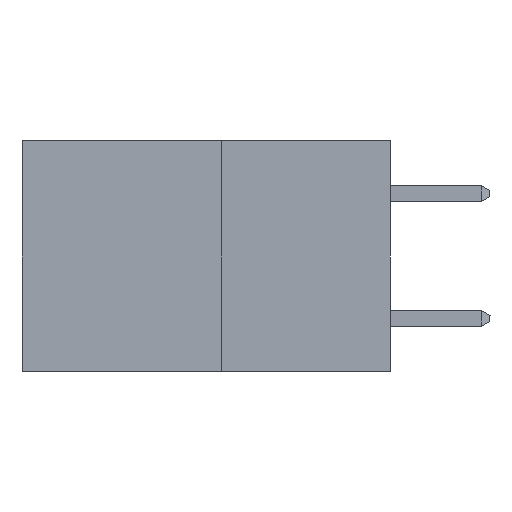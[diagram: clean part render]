
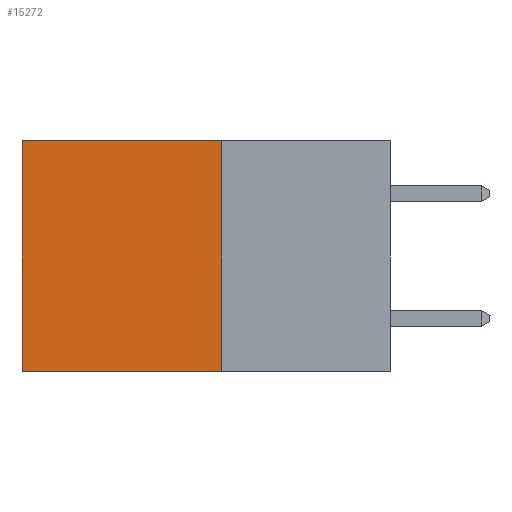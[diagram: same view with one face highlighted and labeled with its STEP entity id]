
A CAD part, left-side view. The second image highlights one B-rep face of the part: STEP entity #15272.
In plain terms, the highlighted planar face has unit normal (-1, 0, 0).
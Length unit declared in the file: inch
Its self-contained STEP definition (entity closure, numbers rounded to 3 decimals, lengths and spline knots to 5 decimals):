
#1228 = VERTEX_POINT ( 'NONE', #15493 ) ;
#1375 = PLANE ( 'NONE',  #30467 ) ;
#1493 = DIRECTION ( 'NONE',  ( 1., 0., 0. ) ) ;
#1712 = VECTOR ( 'NONE', #8613, 39.37008 ) ;
#1733 = VECTOR ( 'NONE', #33003, 39.37008 ) ;
#2395 = CARTESIAN_POINT ( 'NONE',  ( 0.277, 0.59, -0.37 ) ) ;
#2786 = VERTEX_POINT ( 'NONE', #28604 ) ;
#5936 = VECTOR ( 'NONE', #17146, 39.37008 ) ;
#6020 = CARTESIAN_POINT ( 'NONE',  ( 0.277, 0.27, -0.37 ) ) ;
#6703 = LINE ( 'NONE', #16378, #32387 ) ;
#7818 = ORIENTED_EDGE ( 'NONE', *, *, #26788, .F. ) ;
#8156 = ORIENTED_EDGE ( 'NONE', *, *, #24488, .F. ) ;
#8613 = DIRECTION ( 'NONE',  ( 0., 0., -1. ) ) ;
#10356 = ORIENTED_EDGE ( 'NONE', *, *, #28336, .T. ) ;
#12945 = ORIENTED_EDGE ( 'NONE', *, *, #30673, .T. ) ;
#12955 = CARTESIAN_POINT ( 'NONE',  ( 0.277, 0.59, -0.37 ) ) ;
#14595 = CARTESIAN_POINT ( 'NONE',  ( 0.277, 0.27, -0.37 ) ) ;
#14860 = EDGE_LOOP ( 'NONE', ( #12945, #7818, #8156, #10356 ) ) ;
#15272 = ADVANCED_FACE ( 'NONE', ( #21255 ), #1375, .F. ) ;
#15493 = CARTESIAN_POINT ( 'NONE',  ( 0.277, 0.27, 0. ) ) ;
#16360 = VERTEX_POINT ( 'NONE', #12955 ) ;
#16378 = CARTESIAN_POINT ( 'NONE',  ( 0.277, 0.27, 0. ) ) ;
#16700 = CARTESIAN_POINT ( 'NONE',  ( 0.277, 0.27, -0.37 ) ) ;
#17146 = DIRECTION ( 'NONE',  ( 0., 1., 0. ) ) ;
#18817 = VERTEX_POINT ( 'NONE', #19926 ) ;
#19293 = DIRECTION ( 'NONE',  ( 0., 0., -1. ) ) ;
#19463 = LINE ( 'NONE', #14595, #5936 ) ;
#19926 = CARTESIAN_POINT ( 'NONE',  ( 0.277, 0.27, -0.37 ) ) ;
#21255 = FACE_OUTER_BOUND ( 'NONE', #14860, .T. ) ;
#22061 = LINE ( 'NONE', #2395, #1733 ) ;
#24488 = EDGE_CURVE ( 'NONE', #1228, #18817, #28180, .T. ) ;
#26709 = DIRECTION ( 'NONE',  ( 0., 1., 0. ) ) ;
#26788 = EDGE_CURVE ( 'NONE', #18817, #16360, #19463, .T. ) ;
#28180 = LINE ( 'NONE', #6020, #1712 ) ;
#28336 = EDGE_CURVE ( 'NONE', #1228, #2786, #6703, .T. ) ;
#28604 = CARTESIAN_POINT ( 'NONE',  ( 0.277, 0.59, 0. ) ) ;
#30467 = AXIS2_PLACEMENT_3D ( 'NONE', #16700, #1493, #19293 ) ;
#30673 = EDGE_CURVE ( 'NONE', #2786, #16360, #22061, .T. ) ;
#32387 = VECTOR ( 'NONE', #26709, 39.37008 ) ;
#33003 = DIRECTION ( 'NONE',  ( 0., 0., -1. ) ) ;
